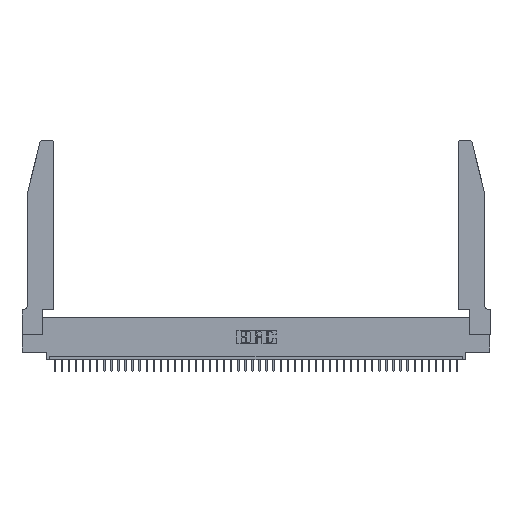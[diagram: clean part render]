
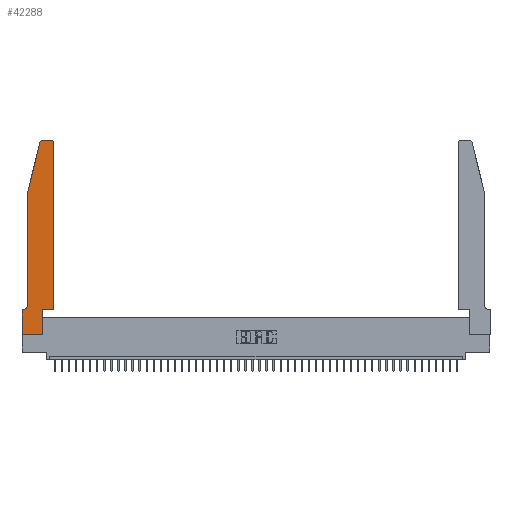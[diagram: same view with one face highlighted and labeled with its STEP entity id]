
A CAD part, top view. The second image highlights one B-rep face of the part: STEP entity #42288.
In plain terms, the highlighted planar face has unit normal (0, 0, 1).
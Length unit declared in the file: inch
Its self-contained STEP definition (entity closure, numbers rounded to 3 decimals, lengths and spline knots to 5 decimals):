
#14 = VERTEX_POINT ( 'NONE', #6731 ) ;
#150 = DIRECTION ( 'NONE',  ( 0., 0., 1. ) ) ;
#290 = LINE ( 'NONE', #45760, #24515 ) ;
#298 = EDGE_CURVE ( 'NONE', #37946, #7661, #19406, .T. ) ;
#711 = CARTESIAN_POINT ( 'NONE',  ( 0.0755, 2., 0.37 ) ) ;
#989 = VECTOR ( 'NONE', #15563, 39.37008 ) ;
#996 = EDGE_CURVE ( 'NONE', #34203, #1236, #2543, .T. ) ;
#1236 = VERTEX_POINT ( 'NONE', #10258 ) ;
#1360 = VECTOR ( 'NONE', #46335, 39.37008 ) ;
#1417 = FACE_OUTER_BOUND ( 'NONE', #26482, .T. ) ;
#1745 = CARTESIAN_POINT ( 'NONE',  ( 0.284, 2.75, 0.37 ) ) ;
#1911 = VECTOR ( 'NONE', #26281, 39.37008 ) ;
#2423 = VECTOR ( 'NONE', #40836, 39.37008 ) ;
#2543 = LINE ( 'NONE', #21255, #1360 ) ;
#2849 = CARTESIAN_POINT ( 'NONE',  ( 0.2865, 0.35, 0.37 ) ) ;
#3002 = DIRECTION ( 'NONE',  ( 0., 1., 0. ) ) ;
#3382 = DIRECTION ( 'NONE',  ( 0., 0., -1. ) ) ;
#3641 = EDGE_CURVE ( 'NONE', #27848, #16838, #40623, .T. ) ;
#4513 = VECTOR ( 'NONE', #45589, 39.37008 ) ;
#4737 = AXIS2_PLACEMENT_3D ( 'NONE', #37265, #30531, #37723 ) ;
#5707 = EDGE_CURVE ( 'NONE', #14, #15329, #36585, .T. ) ;
#5785 = CARTESIAN_POINT ( 'NONE',  ( 0.2605, 2.75, 0.37 ) ) ;
#6548 = DIRECTION ( 'NONE',  ( 1., 0., 0. ) ) ;
#6731 = CARTESIAN_POINT ( 'NONE',  ( 0.0055, 0.35, 0.37 ) ) ;
#6857 = ORIENTED_EDGE ( 'NONE', *, *, #23095, .T. ) ;
#6969 = EDGE_CURVE ( 'NONE', #36654, #38320, #15130, .T. ) ;
#7661 = VERTEX_POINT ( 'NONE', #9280 ) ;
#8033 = LINE ( 'NONE', #711, #1911 ) ;
#8205 = ORIENTED_EDGE ( 'NONE', *, *, #3641, .T. ) ;
#9073 = AXIS2_PLACEMENT_3D ( 'NONE', #35588, #150, #42798 ) ;
#9280 = CARTESIAN_POINT ( 'NONE',  ( 0.4205, 2.75, 0.37 ) ) ;
#10258 = CARTESIAN_POINT ( 'NONE',  ( 0.4505, 0.35, 0.37 ) ) ;
#10826 = DIRECTION ( 'NONE',  ( -1., 0., 0. ) ) ;
#11092 = CARTESIAN_POINT ( 'NONE',  ( 0.2865, 0., 0.37 ) ) ;
#12048 = CARTESIAN_POINT ( 'NONE',  ( 0.0755, 2., 0.37 ) ) ;
#13687 = VERTEX_POINT ( 'NONE', #11092 ) ;
#15130 = LINE ( 'NONE', #31132, #4513 ) ;
#15329 = VERTEX_POINT ( 'NONE', #16334 ) ;
#15563 = DIRECTION ( 'NONE',  ( 0., 1., 0. ) ) ;
#15658 = LINE ( 'NONE', #16246, #24169 ) ;
#16246 = CARTESIAN_POINT ( 'NONE',  ( 0., 0., 0.37 ) ) ;
#16334 = CARTESIAN_POINT ( 'NONE',  ( 0., 0.35, 0.37 ) ) ;
#16838 = VERTEX_POINT ( 'NONE', #38532 ) ;
#17287 = CARTESIAN_POINT ( 'NONE',  ( 0., 0., 0.37 ) ) ;
#18339 = VECTOR ( 'NONE', #3002, 39.37008 ) ;
#19406 = CIRCLE ( 'NONE', #9073, 0.03 ) ;
#19571 = ORIENTED_EDGE ( 'NONE', *, *, #45728, .T. ) ;
#20112 = LINE ( 'NONE', #43458, #989 ) ;
#21255 = CARTESIAN_POINT ( 'NONE',  ( 0.4505, 0.35, 0.37 ) ) ;
#22426 = CARTESIAN_POINT ( 'NONE',  ( 0.4505, 2.72, 0.37 ) ) ;
#23095 = EDGE_CURVE ( 'NONE', #27225, #13687, #15658, .T. ) ;
#24125 = EDGE_CURVE ( 'NONE', #1236, #37946, #20112, .T. ) ;
#24169 = VECTOR ( 'NONE', #45256, 39.37008 ) ;
#24515 = VECTOR ( 'NONE', #30671, 39.37008 ) ;
#24585 = EDGE_CURVE ( 'NONE', #13687, #34203, #45273, .T. ) ;
#25258 = ORIENTED_EDGE ( 'NONE', *, *, #298, .T. ) ;
#26281 = DIRECTION ( 'NONE',  ( -0.239, -0.971, 0. ) ) ;
#26482 = EDGE_LOOP ( 'NONE', ( #31453, #8205, #19571, #40038, #42979, #35972, #35586, #6857, #32511, #32037, #36946, #25258 ) ) ;
#27225 = VERTEX_POINT ( 'NONE', #17287 ) ;
#27789 = LINE ( 'NONE', #5785, #35019 ) ;
#27848 = VERTEX_POINT ( 'NONE', #1745 ) ;
#30531 = DIRECTION ( 'NONE',  ( 0., 0., 1. ) ) ;
#30671 = DIRECTION ( 'NONE',  ( 0., -1., 0. ) ) ;
#31132 = CARTESIAN_POINT ( 'NONE',  ( 0.0755, 2., 0.37 ) ) ;
#31453 = ORIENTED_EDGE ( 'NONE', *, *, #33793, .T. ) ;
#32037 = ORIENTED_EDGE ( 'NONE', *, *, #996, .T. ) ;
#32511 = ORIENTED_EDGE ( 'NONE', *, *, #24585, .T. ) ;
#33793 = EDGE_CURVE ( 'NONE', #7661, #27848, #27789, .T. ) ;
#34203 = VERTEX_POINT ( 'NONE', #44965 ) ;
#35019 = VECTOR ( 'NONE', #41643, 39.37008 ) ;
#35586 = ORIENTED_EDGE ( 'NONE', *, *, #44738, .T. ) ;
#35588 = CARTESIAN_POINT ( 'NONE',  ( 0.4205, 2.72, 0.37 ) ) ;
#35972 = ORIENTED_EDGE ( 'NONE', *, *, #5707, .T. ) ;
#36585 = LINE ( 'NONE', #37228, #2423 ) ;
#36654 = VERTEX_POINT ( 'NONE', #12048 ) ;
#36946 = ORIENTED_EDGE ( 'NONE', *, *, #24125, .T. ) ;
#37228 = CARTESIAN_POINT ( 'NONE',  ( 0.0755, 0.35, 0.37 ) ) ;
#37265 = CARTESIAN_POINT ( 'NONE',  ( 0., 0.35, 0.37 ) ) ;
#37723 = DIRECTION ( 'NONE',  ( 1., 0., 0. ) ) ;
#37946 = VERTEX_POINT ( 'NONE', #22426 ) ;
#38320 = VERTEX_POINT ( 'NONE', #40315 ) ;
#38532 = CARTESIAN_POINT ( 'NONE',  ( 0.25487, 2.72718, 0.37 ) ) ;
#38908 = CARTESIAN_POINT ( 'NONE',  ( 0.0055, 0.42, 0.37 ) ) ;
#40038 = ORIENTED_EDGE ( 'NONE', *, *, #6969, .T. ) ;
#40315 = CARTESIAN_POINT ( 'NONE',  ( 0.0755, 0.42, 0.37 ) ) ;
#40623 = CIRCLE ( 'NONE', #42321, 0.03 ) ;
#40836 = DIRECTION ( 'NONE',  ( -1., 0., 0. ) ) ;
#41643 = DIRECTION ( 'NONE',  ( -1., 0., 0. ) ) ;
#41796 = CARTESIAN_POINT ( 'NONE',  ( 0.284, 2.72, 0.37 ) ) ;
#42288 = ADVANCED_FACE ( 'NONE', ( #1417 ), #44818, .T. ) ;
#42321 = AXIS2_PLACEMENT_3D ( 'NONE', #41796, #45885, #6548 ) ;
#42798 = DIRECTION ( 'NONE',  ( 1., 0., 0. ) ) ;
#42979 = ORIENTED_EDGE ( 'NONE', *, *, #45533, .T. ) ;
#43458 = CARTESIAN_POINT ( 'NONE',  ( 0.4505, 0.35, 0.37 ) ) ;
#43569 = AXIS2_PLACEMENT_3D ( 'NONE', #38908, #3382, #10826 ) ;
#44548 = CIRCLE ( 'NONE', #43569, 0.07 ) ;
#44738 = EDGE_CURVE ( 'NONE', #15329, #27225, #290, .T. ) ;
#44818 = PLANE ( 'NONE',  #4737 ) ;
#44965 = CARTESIAN_POINT ( 'NONE',  ( 0.2865, 0.35, 0.37 ) ) ;
#45256 = DIRECTION ( 'NONE',  ( 1., 0., 0. ) ) ;
#45273 = LINE ( 'NONE', #2849, #18339 ) ;
#45533 = EDGE_CURVE ( 'NONE', #38320, #14, #44548, .T. ) ;
#45589 = DIRECTION ( 'NONE',  ( 0., -1., 0. ) ) ;
#45728 = EDGE_CURVE ( 'NONE', #16838, #36654, #8033, .T. ) ;
#45760 = CARTESIAN_POINT ( 'NONE',  ( 0., 0., 0.37 ) ) ;
#45885 = DIRECTION ( 'NONE',  ( 0., 0., 1. ) ) ;
#46335 = DIRECTION ( 'NONE',  ( 1., 0., 0. ) ) ;
